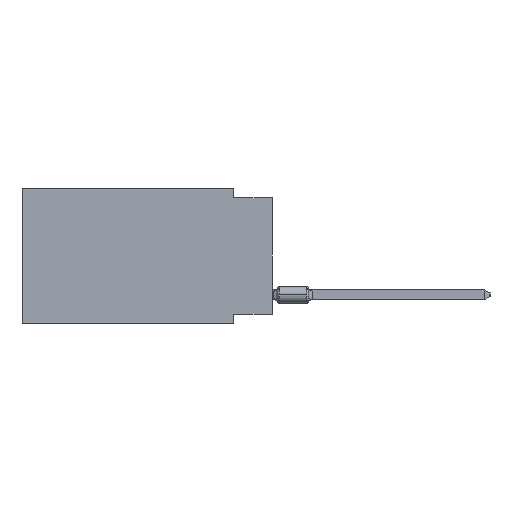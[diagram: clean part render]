
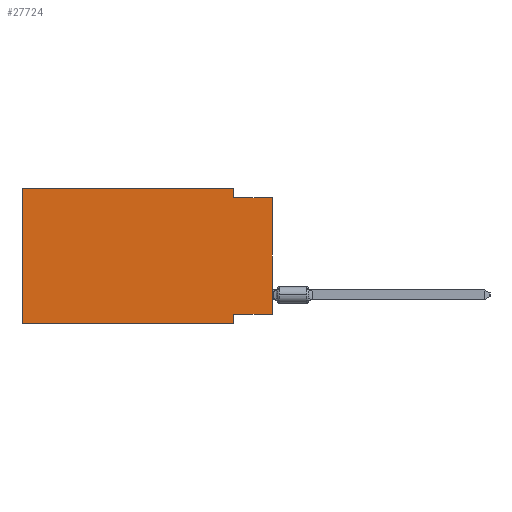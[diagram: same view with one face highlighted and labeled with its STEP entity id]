
A CAD part, left-side view. The second image highlights one B-rep face of the part: STEP entity #27724.
In plain terms, the highlighted planar face has unit normal (-1, 0, 0).
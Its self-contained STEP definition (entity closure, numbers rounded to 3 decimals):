
#339 = VECTOR ( 'NONE', #3964, 1000. ) ;
#3546 = LINE ( 'NONE', #38984, #8998 ) ;
#3964 = DIRECTION ( 'NONE',  ( 0., 0., -1. ) ) ;
#4079 = CARTESIAN_POINT ( 'NONE',  ( 0., 0., 0. ) ) ;
#4624 = CARTESIAN_POINT ( 'NONE',  ( 0., 2.54, -8.89 ) ) ;
#5140 = EDGE_CURVE ( 'NONE', #15753, #10876, #9768, .T. ) ;
#6399 = CARTESIAN_POINT ( 'NONE',  ( 0., 2.54, 0. ) ) ;
#6930 = EDGE_CURVE ( 'NONE', #53380, #35666, #27762, .T. ) ;
#8319 = EDGE_CURVE ( 'NONE', #35666, #18298, #11176, .T. ) ;
#8998 = VECTOR ( 'NONE', #63695, 1000. ) ;
#9315 = ORIENTED_EDGE ( 'NONE', *, *, #17452, .T. ) ;
#9768 = LINE ( 'NONE', #28811, #26657 ) ;
#9863 = EDGE_CURVE ( 'NONE', #15753, #40132, #28250, .T. ) ;
#10193 = CARTESIAN_POINT ( 'NONE',  ( 0., 0., -0.635 ) ) ;
#10876 = VERTEX_POINT ( 'NONE', #51936 ) ;
#11176 = LINE ( 'NONE', #10193, #37605 ) ;
#12883 = VECTOR ( 'NONE', #32450, 1000. ) ;
#13510 = EDGE_LOOP ( 'NONE', ( #9315, #45128, #63939, #44515, #27883, #39507, #49203, #36892 ) ) ;
#15753 = VERTEX_POINT ( 'NONE', #46885 ) ;
#17452 = EDGE_CURVE ( 'NONE', #28784, #18298, #19798, .T. ) ;
#17563 = VECTOR ( 'NONE', #40181, 1000. ) ;
#17883 = DIRECTION ( 'NONE',  ( 0., -1., 0. ) ) ;
#18298 = VERTEX_POINT ( 'NONE', #59130 ) ;
#19798 = LINE ( 'NONE', #4079, #17563 ) ;
#21274 = CARTESIAN_POINT ( 'NONE',  ( 0., 16.383, 0. ) ) ;
#24476 = DIRECTION ( 'NONE',  ( 0., 0., 1. ) ) ;
#25950 = DIRECTION ( 'NONE',  ( 0., -1., 0. ) ) ;
#26657 = VECTOR ( 'NONE', #24476, 1000. ) ;
#26936 = LINE ( 'NONE', #21274, #42385 ) ;
#27724 = ADVANCED_FACE ( 'NONE', ( #35245 ), #55607, .F. ) ;
#27762 = LINE ( 'NONE', #6399, #12883 ) ;
#27883 = ORIENTED_EDGE ( 'NONE', *, *, #5140, .F. ) ;
#28250 = LINE ( 'NONE', #59288, #40020 ) ;
#28784 = VERTEX_POINT ( 'NONE', #65903 ) ;
#28811 = CARTESIAN_POINT ( 'NONE',  ( 0., 16.383, 0. ) ) ;
#31576 = DIRECTION ( 'NONE',  ( 0., -1., 0. ) ) ;
#31888 = EDGE_CURVE ( 'NONE', #10876, #53380, #26936, .T. ) ;
#32450 = DIRECTION ( 'NONE',  ( 0., 0., -1. ) ) ;
#35245 = FACE_OUTER_BOUND ( 'NONE', #13510, .T. ) ;
#35572 = CARTESIAN_POINT ( 'NONE',  ( 0., 16.383, 0. ) ) ;
#35666 = VERTEX_POINT ( 'NONE', #53739 ) ;
#35711 = LINE ( 'NONE', #4624, #339 ) ;
#36274 = CARTESIAN_POINT ( 'NONE',  ( 0., 2.54, -8.89 ) ) ;
#36892 = ORIENTED_EDGE ( 'NONE', *, *, #39080, .F. ) ;
#37605 = VECTOR ( 'NONE', #31576, 1000. ) ;
#38984 = CARTESIAN_POINT ( 'NONE',  ( 0., 0., -8.255 ) ) ;
#39080 = EDGE_CURVE ( 'NONE', #28784, #55186, #3546, .T. ) ;
#39507 = ORIENTED_EDGE ( 'NONE', *, *, #9863, .T. ) ;
#39599 = EDGE_CURVE ( 'NONE', #55186, #40132, #35711, .T. ) ;
#40020 = VECTOR ( 'NONE', #17883, 1000. ) ;
#40132 = VERTEX_POINT ( 'NONE', #36274 ) ;
#40181 = DIRECTION ( 'NONE',  ( 0., 0., 1. ) ) ;
#42385 = VECTOR ( 'NONE', #25950, 1000. ) ;
#43338 = CARTESIAN_POINT ( 'NONE',  ( 0., 2.54, -8.255 ) ) ;
#44515 = ORIENTED_EDGE ( 'NONE', *, *, #31888, .F. ) ;
#45128 = ORIENTED_EDGE ( 'NONE', *, *, #8319, .F. ) ;
#45920 = DIRECTION ( 'NONE',  ( 1., 0., 0. ) ) ;
#46592 = DIRECTION ( 'NONE',  ( 0., 0., -1. ) ) ;
#46885 = CARTESIAN_POINT ( 'NONE',  ( 0., 16.383, -8.89 ) ) ;
#49203 = ORIENTED_EDGE ( 'NONE', *, *, #39599, .F. ) ;
#51936 = CARTESIAN_POINT ( 'NONE',  ( 0., 16.383, 0. ) ) ;
#53380 = VERTEX_POINT ( 'NONE', #65023 ) ;
#53739 = CARTESIAN_POINT ( 'NONE',  ( 0., 2.54, -0.635 ) ) ;
#54268 = AXIS2_PLACEMENT_3D ( 'NONE', #35572, #45920, #46592 ) ;
#55186 = VERTEX_POINT ( 'NONE', #43338 ) ;
#55607 = PLANE ( 'NONE',  #54268 ) ;
#59130 = CARTESIAN_POINT ( 'NONE',  ( 0., 0., -0.635 ) ) ;
#59288 = CARTESIAN_POINT ( 'NONE',  ( 0., 16.383, -8.89 ) ) ;
#63695 = DIRECTION ( 'NONE',  ( 0., 1., 0. ) ) ;
#63939 = ORIENTED_EDGE ( 'NONE', *, *, #6930, .F. ) ;
#65023 = CARTESIAN_POINT ( 'NONE',  ( 0., 2.54, 0. ) ) ;
#65903 = CARTESIAN_POINT ( 'NONE',  ( 0., 0., -8.255 ) ) ;
